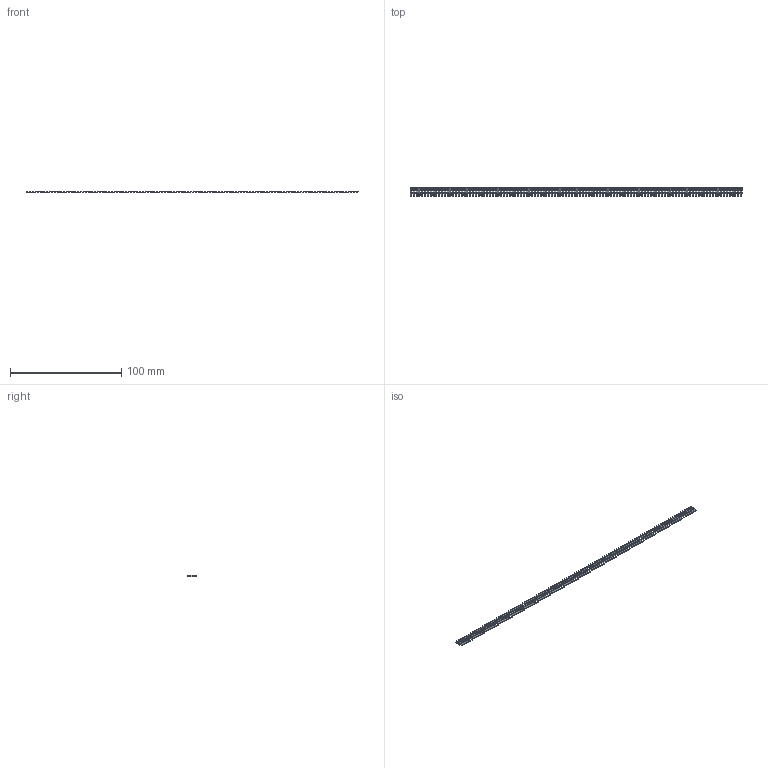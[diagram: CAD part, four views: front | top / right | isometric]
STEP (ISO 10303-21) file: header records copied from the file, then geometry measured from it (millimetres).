
FILE_DESCRIPTION (( 'STEP AP203' ), '1' );
FILE_NAME ('106-118-253-100.STEP', '2020-04-16T23:42:39', ( '' ), ( '' ), 'SwSTEP 2.0', 'SolidWorks 2016', '' );
FILE_SCHEMA (( 'CONFIG_CONTROL_DESIGN' ));
Length unit declared in the file: inch
Products named in the file (2): 100-290-001_100-290-253; 106-118-253-100
Assembly tree (118 placements, depth 2):
  106-118-253-100
    100-290-001_100-290-253  x118
Bounding box: 298.98 x 7.62 x 1.8 mm (x, y, z)
Volume: 651.1 mm3; surface area: 4060 mm2
Topology: 118 solids, 118 shells, 2360 faces, 6372 edges, 4248 vertices
Faces by surface type: plane 2242, cylinder 118
Entity records: 4564 total; most frequent: DIRECTION 338, DATE_AND_TIME 246, LOCAL_TIME 246, CALENDAR_DATE 246, COORDINATED_UNIVERSAL_TIME_OFFSET 246, CARTESIAN_POINT 231, AXIS2_PLACEMENT_3D 143, PERSON_AND_ORGANIZATION 134
